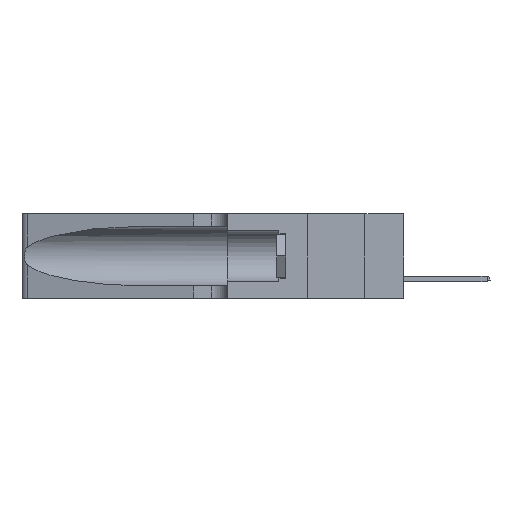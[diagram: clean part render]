
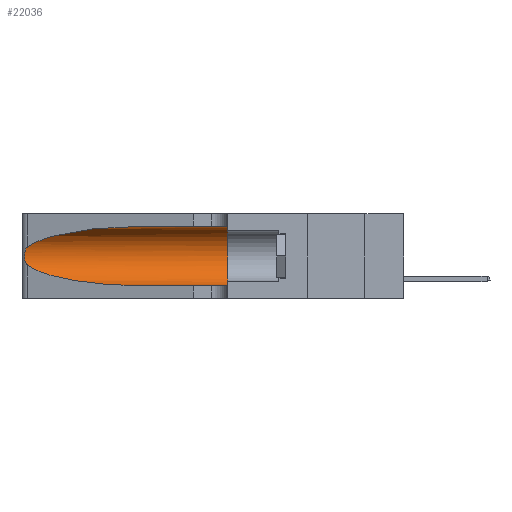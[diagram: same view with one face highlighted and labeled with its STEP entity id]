
A CAD part, left-side view. The second image highlights one B-rep face of the part: STEP entity #22036.
In plain terms, the highlighted cylindrical face has radius 3.308 mm (diameter 6.617 mm), a partial arc.
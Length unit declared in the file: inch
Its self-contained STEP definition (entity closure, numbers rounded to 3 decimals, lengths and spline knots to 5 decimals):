
#139 = CYLINDRICAL_SURFACE ( 'NONE', #10967, 0.13025 ) ;
#211 = VERTEX_POINT ( 'NONE', #31522 ) ;
#811 = CARTESIAN_POINT ( 'NONE',  ( 0.1305, 1.61858, 0.185 ) ) ;
#1405 = AXIS2_PLACEMENT_3D ( 'NONE', #23817, #17560, #17435 ) ;
#2065 = B_SPLINE_CURVE_WITH_KNOTS ( 'NONE', 3,
 ( #25106, #27892, #31065, #30933, #2518, #11876, #28036, #15504, #8791, #12165, #34455, #15371, #37664, #9075 ),
 .UNSPECIFIED., .F., .F.,
 ( 4, 2, 2, 2, 2, 2, 4 ),
 ( 0., 0.00027, 0.00053, 0.00107, 0.0016, 0.00187, 0.00214 ),
 .UNSPECIFIED. ) ;
#2166 = CARTESIAN_POINT ( 'NONE',  ( 0.25487, 1.22718, 0.14631 ) ) ;
#2518 = CARTESIAN_POINT ( 'NONE',  ( 0.25854, 1.2359, 0.20912 ) ) ;
#2700 = CARTESIAN_POINT ( 'NONE',  ( 0.1305, 0.35, 0.31525 ) ) ;
#2926 = ORIENTED_EDGE ( 'NONE', *, *, #38049, .T. ) ;
#4664 = VERTEX_POINT ( 'NONE', #18947 ) ;
#5467 = CARTESIAN_POINT ( 'NONE',  ( 0.1305, 0.72297, 0.31525 ) ) ;
#5537 = CARTESIAN_POINT ( 'NONE',  ( 0.2373, 1.15595, 0.08982 ) ) ;
#5872 = VERTEX_POINT ( 'NONE', #37452 ) ;
#6938 = LINE ( 'NONE', #36100, #40347 ) ;
#6985 = DIRECTION ( 'NONE',  ( 0., -1., 0. ) ) ;
#7663 =( BOUNDED_CURVE ( )  B_SPLINE_CURVE ( 3, ( #5467, #15100, #8371, #37548 ),
 .UNSPECIFIED., .F., .F. ) 
 B_SPLINE_CURVE_WITH_KNOTS ( ( 4, 4 ),
 ( 1.5708, 2.84003 ),
 .UNSPECIFIED. ) 
 CURVE ( )  GEOMETRIC_REPRESENTATION_ITEM ( )  RATIONAL_B_SPLINE_CURVE ( ( 1., 0.87, 0.87, 1. ) ) 
 REPRESENTATION_ITEM ( '' )  );
#7775 = EDGE_LOOP ( 'NONE', ( #32778, #22898, #17021, #2926, #9316, #16480 ) ) ;
#8371 = CARTESIAN_POINT ( 'NONE',  ( 0.2373, 1.15595, 0.28018 ) ) ;
#8791 = CARTESIAN_POINT ( 'NONE',  ( 0.26017, 1.23833, 0.17102 ) ) ;
#9075 = CARTESIAN_POINT ( 'NONE',  ( 0.25487, 1.22718, 0.14631 ) ) ;
#9316 = ORIENTED_EDGE ( 'NONE', *, *, #25542, .F. ) ;
#9672 = FACE_OUTER_BOUND ( 'NONE', #7775, .T. ) ;
#10967 = AXIS2_PLACEMENT_3D ( 'NONE', #811, #6985, #29042 ) ;
#11876 = CARTESIAN_POINT ( 'NONE',  ( 0.26018, 1.23835, 0.19895 ) ) ;
#12165 = CARTESIAN_POINT ( 'NONE',  ( 0.25856, 1.23593, 0.16098 ) ) ;
#13666 = EDGE_CURVE ( 'NONE', #33633, #17285, #21461, .T. ) ;
#14089 = DIRECTION ( 'NONE',  ( 0., -1., 0. ) ) ;
#15100 = CARTESIAN_POINT ( 'NONE',  ( 0.18966, 0.96281, 0.31525 ) ) ;
#15371 = CARTESIAN_POINT ( 'NONE',  ( 0.25639, 1.23186, 0.15144 ) ) ;
#15504 = CARTESIAN_POINT ( 'NONE',  ( 0.26075, 1.23896, 0.178 ) ) ;
#15680 = VERTEX_POINT ( 'NONE', #27913 ) ;
#16480 = ORIENTED_EDGE ( 'NONE', *, *, #13666, .F. ) ;
#17021 = ORIENTED_EDGE ( 'NONE', *, *, #30688, .T. ) ;
#17285 = VERTEX_POINT ( 'NONE', #2700 ) ;
#17435 = DIRECTION ( 'NONE',  ( 0., 0., 1. ) ) ;
#17560 = DIRECTION ( 'NONE',  ( 0., 1., 0. ) ) ;
#18735 = EDGE_CURVE ( 'NONE', #4664, #211, #2065, .T. ) ;
#18947 = CARTESIAN_POINT ( 'NONE',  ( 0.25487, 1.22718, 0.22369 ) ) ;
#20130 = DIRECTION ( 'NONE',  ( 0., -1., 0. ) ) ;
#21461 = LINE ( 'NONE', #39173, #30364 ) ;
#22036 = ADVANCED_FACE ( 'NONE', ( #9672 ), #139, .F. ) ;
#22898 = ORIENTED_EDGE ( 'NONE', *, *, #18735, .T. ) ;
#23817 = CARTESIAN_POINT ( 'NONE',  ( 0.1305, 0.35, 0.185 ) ) ;
#25106 = CARTESIAN_POINT ( 'NONE',  ( 0.25487, 1.22718, 0.22369 ) ) ;
#25542 = EDGE_CURVE ( 'NONE', #17285, #15680, #29038, .T. ) ;
#26917 = EDGE_CURVE ( 'NONE', #33633, #4664, #7663, .T. ) ;
#27892 = CARTESIAN_POINT ( 'NONE',  ( 0.25555, 1.22994, 0.2215 ) ) ;
#27913 = CARTESIAN_POINT ( 'NONE',  ( 0.1305, 0.35, 0.05475 ) ) ;
#28036 = CARTESIAN_POINT ( 'NONE',  ( 0.26075, 1.23896, 0.19203 ) ) ;
#29038 = CIRCLE ( 'NONE', #1405, 0.13025 ) ;
#29042 = DIRECTION ( 'NONE',  ( 0., 0., -1. ) ) ;
#30364 = VECTOR ( 'NONE', #14089, 39.37008 ) ;
#30688 = EDGE_CURVE ( 'NONE', #211, #5872, #34302, .T. ) ;
#30873 = CARTESIAN_POINT ( 'NONE',  ( 0.18966, 0.96281, 0.05475 ) ) ;
#30933 = CARTESIAN_POINT ( 'NONE',  ( 0.25787, 1.23484, 0.2124 ) ) ;
#31065 = CARTESIAN_POINT ( 'NONE',  ( 0.25639, 1.23184, 0.21858 ) ) ;
#31522 = CARTESIAN_POINT ( 'NONE',  ( 0.25487, 1.22718, 0.14631 ) ) ;
#32778 = ORIENTED_EDGE ( 'NONE', *, *, #26917, .T. ) ;
#33633 = VERTEX_POINT ( 'NONE', #38551 ) ;
#33975 = CARTESIAN_POINT ( 'NONE',  ( 0.1305, 0.72297, 0.05475 ) ) ;
#34302 =( BOUNDED_CURVE ( )  B_SPLINE_CURVE ( 3, ( #2166, #5537, #30873, #33975 ),
 .UNSPECIFIED., .F., .F. ) 
 B_SPLINE_CURVE_WITH_KNOTS ( ( 4, 4 ),
 ( 3.44316, 4.71239 ),
 .UNSPECIFIED. ) 
 CURVE ( )  GEOMETRIC_REPRESENTATION_ITEM ( )  RATIONAL_B_SPLINE_CURVE ( ( 1., 0.87, 0.87, 1. ) ) 
 REPRESENTATION_ITEM ( '' )  );
#34455 = CARTESIAN_POINT ( 'NONE',  ( 0.25789, 1.23486, 0.15765 ) ) ;
#36100 = CARTESIAN_POINT ( 'NONE',  ( 0.1305, 1.61858, 0.05475 ) ) ;
#37452 = CARTESIAN_POINT ( 'NONE',  ( 0.1305, 0.72297, 0.05475 ) ) ;
#37548 = CARTESIAN_POINT ( 'NONE',  ( 0.25487, 1.22718, 0.22369 ) ) ;
#37664 = CARTESIAN_POINT ( 'NONE',  ( 0.25555, 1.22993, 0.14849 ) ) ;
#38049 = EDGE_CURVE ( 'NONE', #5872, #15680, #6938, .T. ) ;
#38551 = CARTESIAN_POINT ( 'NONE',  ( 0.1305, 0.72297, 0.31525 ) ) ;
#39173 = CARTESIAN_POINT ( 'NONE',  ( 0.1305, 1.61858, 0.31525 ) ) ;
#40347 = VECTOR ( 'NONE', #20130, 39.37008 ) ;
